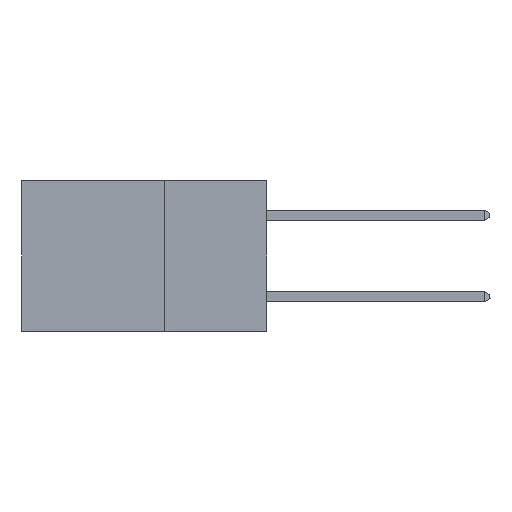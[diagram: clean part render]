
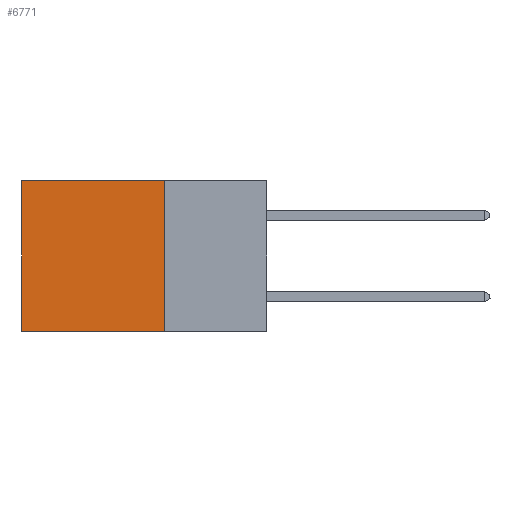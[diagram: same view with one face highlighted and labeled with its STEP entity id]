
A CAD part, left-side view. The second image highlights one B-rep face of the part: STEP entity #6771.
In plain terms, the highlighted planar face has unit normal (-1, 0, 0).
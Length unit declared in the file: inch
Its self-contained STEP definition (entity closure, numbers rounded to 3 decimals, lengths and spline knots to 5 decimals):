
#295 = CARTESIAN_POINT ( 'NONE',  ( 0.2875, 0.6, 0. ) ) ;
#460 = DIRECTION ( 'NONE',  ( 0., 0., -1. ) ) ;
#1760 = LINE ( 'NONE', #5277, #9842 ) ;
#3008 = EDGE_CURVE ( 'NONE', #17549, #9008, #7904, .T. ) ;
#3710 = ORIENTED_EDGE ( 'NONE', *, *, #12721, .T. ) ;
#4764 = PLANE ( 'NONE',  #18084 ) ;
#5238 = CARTESIAN_POINT ( 'NONE',  ( 0.2875, 0.6, -0.37 ) ) ;
#5277 = CARTESIAN_POINT ( 'NONE',  ( 0.2875, 0.25, 0. ) ) ;
#6066 = EDGE_LOOP ( 'NONE', ( #3710, #10327, #15166, #8345 ) ) ;
#6771 = ADVANCED_FACE ( 'NONE', ( #11020 ), #4764, .F. ) ;
#7374 = DIRECTION ( 'NONE',  ( 0., 0., -1. ) ) ;
#7383 = LINE ( 'NONE', #295, #12364 ) ;
#7571 = CARTESIAN_POINT ( 'NONE',  ( 0.2875, 0.25, 0. ) ) ;
#7904 = LINE ( 'NONE', #15897, #16270 ) ;
#7905 = CARTESIAN_POINT ( 'NONE',  ( 0.2875, 0.25, -0.37 ) ) ;
#8345 = ORIENTED_EDGE ( 'NONE', *, *, #8428, .T. ) ;
#8428 = EDGE_CURVE ( 'NONE', #17549, #12575, #1760, .T. ) ;
#9008 = VERTEX_POINT ( 'NONE', #7905 ) ;
#9842 = VECTOR ( 'NONE', #15169, 39.37008 ) ;
#10327 = ORIENTED_EDGE ( 'NONE', *, *, #14815, .F. ) ;
#10501 = DIRECTION ( 'NONE',  ( 1., 0., 0. ) ) ;
#10727 = VERTEX_POINT ( 'NONE', #5238 ) ;
#11020 = FACE_OUTER_BOUND ( 'NONE', #6066, .T. ) ;
#11633 = CARTESIAN_POINT ( 'NONE',  ( 0.2875, 0.25, 0. ) ) ;
#12364 = VECTOR ( 'NONE', #13263, 39.37008 ) ;
#12463 = DIRECTION ( 'NONE',  ( 0., 1., 0. ) ) ;
#12515 = LINE ( 'NONE', #15048, #18136 ) ;
#12575 = VERTEX_POINT ( 'NONE', #12735 ) ;
#12721 = EDGE_CURVE ( 'NONE', #12575, #10727, #7383, .T. ) ;
#12735 = CARTESIAN_POINT ( 'NONE',  ( 0.2875, 0.6, 0. ) ) ;
#13263 = DIRECTION ( 'NONE',  ( 0., 0., -1. ) ) ;
#14815 = EDGE_CURVE ( 'NONE', #9008, #10727, #12515, .T. ) ;
#15048 = CARTESIAN_POINT ( 'NONE',  ( 0.2875, 0.25, -0.37 ) ) ;
#15166 = ORIENTED_EDGE ( 'NONE', *, *, #3008, .F. ) ;
#15169 = DIRECTION ( 'NONE',  ( 0., 1., 0. ) ) ;
#15897 = CARTESIAN_POINT ( 'NONE',  ( 0.2875, 0.25, 0. ) ) ;
#16270 = VECTOR ( 'NONE', #7374, 39.37008 ) ;
#17549 = VERTEX_POINT ( 'NONE', #11633 ) ;
#18084 = AXIS2_PLACEMENT_3D ( 'NONE', #7571, #10501, #460 ) ;
#18136 = VECTOR ( 'NONE', #12463, 39.37008 ) ;
